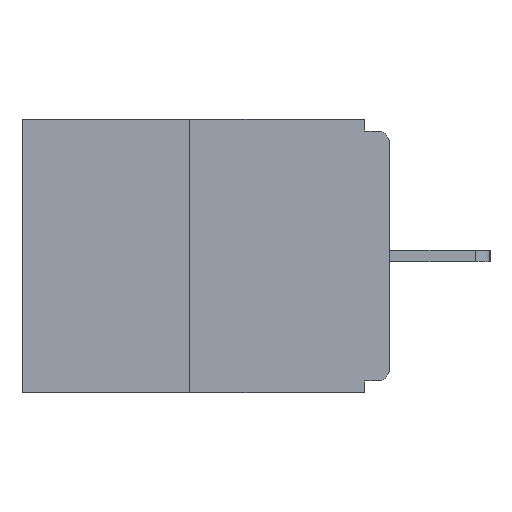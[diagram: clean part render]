
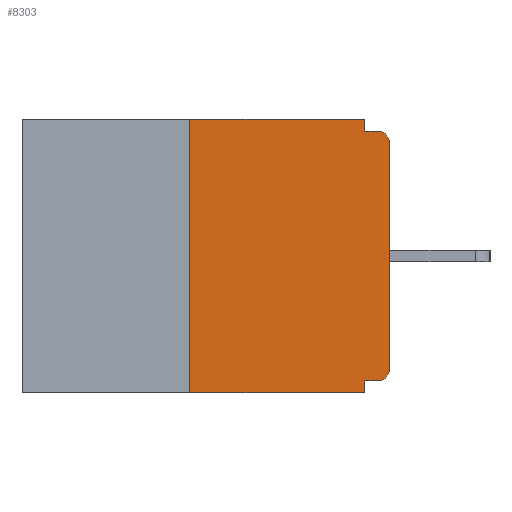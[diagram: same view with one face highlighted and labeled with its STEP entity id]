
A CAD part, left-side view. The second image highlights one B-rep face of the part: STEP entity #8303.
In plain terms, the highlighted planar face has unit normal (-1, 0, 0).
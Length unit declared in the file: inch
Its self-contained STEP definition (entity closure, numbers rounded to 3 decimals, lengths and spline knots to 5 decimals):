
#820 = VERTEX_POINT ( 'NONE', #8225 ) ;
#837 = LINE ( 'NONE', #11827, #17654 ) ;
#932 = VECTOR ( 'NONE', #15600, 39.37008 ) ;
#1601 = ORIENTED_EDGE ( 'NONE', *, *, #10227, .T. ) ;
#2636 = LINE ( 'NONE', #14006, #5194 ) ;
#3064 = EDGE_CURVE ( 'NONE', #14530, #14512, #12996, .T. ) ;
#3083 = VECTOR ( 'NONE', #16883, 39.37008 ) ;
#3139 = EDGE_CURVE ( 'NONE', #20137, #10788, #2636, .T. ) ;
#3146 = ORIENTED_EDGE ( 'NONE', *, *, #3064, .T. ) ;
#3280 = DIRECTION ( 'NONE',  ( 0., 1., 0. ) ) ;
#3359 = DIRECTION ( 'NONE',  ( 0., 0., -1. ) ) ;
#4094 = CARTESIAN_POINT ( 'NONE',  ( 0., 0.46, -0.343 ) ) ;
#4620 = ORIENTED_EDGE ( 'NONE', *, *, #8521, .F. ) ;
#5000 = CARTESIAN_POINT ( 'NONE',  ( 0., 0.015, -0.328 ) ) ;
#5194 = VECTOR ( 'NONE', #19680, 39.37008 ) ;
#5853 = ORIENTED_EDGE ( 'NONE', *, *, #8790, .F. ) ;
#5924 = CARTESIAN_POINT ( 'NONE',  ( 0., 0.015, -0.313 ) ) ;
#6240 = DIRECTION ( 'NONE',  ( -1., 0., 0. ) ) ;
#6523 = ORIENTED_EDGE ( 'NONE', *, *, #3139, .F. ) ;
#6642 = CARTESIAN_POINT ( 'NONE',  ( 0., 0.015, -0.015 ) ) ;
#6735 = LINE ( 'NONE', #13248, #15952 ) ;
#7160 = VECTOR ( 'NONE', #17291, 39.37008 ) ;
#7261 = ORIENTED_EDGE ( 'NONE', *, *, #9357, .T. ) ;
#7891 = DIRECTION ( 'NONE',  ( 1., 0., 0. ) ) ;
#8225 = CARTESIAN_POINT ( 'NONE',  ( 0., 0., -0.03 ) ) ;
#8303 = ADVANCED_FACE ( 'NONE', ( #14293 ), #17512, .F. ) ;
#8521 = EDGE_CURVE ( 'NONE', #13873, #20323, #6735, .T. ) ;
#8570 = ORIENTED_EDGE ( 'NONE', *, *, #16606, .F. ) ;
#8790 = EDGE_CURVE ( 'NONE', #14530, #13873, #19564, .T. ) ;
#8847 = CARTESIAN_POINT ( 'NONE',  ( 0., 0.015, -0.03 ) ) ;
#9051 = CARTESIAN_POINT ( 'NONE',  ( 0., 0.031, -0.015 ) ) ;
#9179 = VERTEX_POINT ( 'NONE', #11433 ) ;
#9357 = EDGE_CURVE ( 'NONE', #820, #13714, #9615, .T. ) ;
#9615 = CIRCLE ( 'NONE', #20498, 0.015 ) ;
#10192 = VECTOR ( 'NONE', #16872, 39.37008 ) ;
#10227 = EDGE_CURVE ( 'NONE', #14512, #820, #15177, .T. ) ;
#10382 = CARTESIAN_POINT ( 'NONE',  ( 0., 0., -0.015 ) ) ;
#10443 = EDGE_LOOP ( 'NONE', ( #8570, #11924, #17561, #4620, #5853, #3146, #1601, #7261, #17327, #6523 ) ) ;
#10504 = VECTOR ( 'NONE', #3280, 39.37008 ) ;
#10788 = VERTEX_POINT ( 'NONE', #9051 ) ;
#10869 = CARTESIAN_POINT ( 'NONE',  ( 0., 0.46, 0. ) ) ;
#10878 = CARTESIAN_POINT ( 'NONE',  ( 0., 0.25, -0.343 ) ) ;
#11433 = CARTESIAN_POINT ( 'NONE',  ( 0., 0.25, 0. ) ) ;
#11827 = CARTESIAN_POINT ( 'NONE',  ( 0., 0.25, 0. ) ) ;
#11924 = ORIENTED_EDGE ( 'NONE', *, *, #12956, .F. ) ;
#11957 = DIRECTION ( 'NONE',  ( 0., 0., -1. ) ) ;
#11999 = EDGE_CURVE ( 'NONE', #10788, #13714, #18597, .T. ) ;
#12189 = AXIS2_PLACEMENT_3D ( 'NONE', #16027, #7891, #3359 ) ;
#12192 = CARTESIAN_POINT ( 'NONE',  ( 0., 0., 0. ) ) ;
#12247 = DIRECTION ( 'NONE',  ( 0., 0., 1. ) ) ;
#12744 = DIRECTION ( 'NONE',  ( 0., 0., -1. ) ) ;
#12780 = CARTESIAN_POINT ( 'NONE',  ( 0., 0.031, -0.343 ) ) ;
#12956 = EDGE_CURVE ( 'NONE', #17377, #9179, #837, .T. ) ;
#12996 = CIRCLE ( 'NONE', #15727, 0.015 ) ;
#13248 = CARTESIAN_POINT ( 'NONE',  ( 0., 0.031, -0.343 ) ) ;
#13714 = VERTEX_POINT ( 'NONE', #6642 ) ;
#13737 = EDGE_CURVE ( 'NONE', #17377, #20323, #15579, .T. ) ;
#13873 = VERTEX_POINT ( 'NONE', #19099 ) ;
#14006 = CARTESIAN_POINT ( 'NONE',  ( 0., 0.031, 0. ) ) ;
#14293 = FACE_OUTER_BOUND ( 'NONE', #10443, .T. ) ;
#14512 = VERTEX_POINT ( 'NONE', #17894 ) ;
#14530 = VERTEX_POINT ( 'NONE', #5000 ) ;
#15049 = DIRECTION ( 'NONE',  ( -1., 0., 0. ) ) ;
#15177 = LINE ( 'NONE', #12192, #3083 ) ;
#15579 = LINE ( 'NONE', #4094, #10192 ) ;
#15600 = DIRECTION ( 'NONE',  ( 0., -1., 0. ) ) ;
#15727 = AXIS2_PLACEMENT_3D ( 'NONE', #5924, #6240, #12744 ) ;
#15952 = VECTOR ( 'NONE', #19749, 39.37008 ) ;
#16027 = CARTESIAN_POINT ( 'NONE',  ( 0., 0.46, 0. ) ) ;
#16269 = CARTESIAN_POINT ( 'NONE',  ( 0., 0., -0.328 ) ) ;
#16606 = EDGE_CURVE ( 'NONE', #9179, #20137, #19199, .T. ) ;
#16872 = DIRECTION ( 'NONE',  ( 0., -1., 0. ) ) ;
#16883 = DIRECTION ( 'NONE',  ( 0., 0., 1. ) ) ;
#17291 = DIRECTION ( 'NONE',  ( 0., -1., 0. ) ) ;
#17327 = ORIENTED_EDGE ( 'NONE', *, *, #11999, .F. ) ;
#17377 = VERTEX_POINT ( 'NONE', #10878 ) ;
#17512 = PLANE ( 'NONE',  #12189 ) ;
#17561 = ORIENTED_EDGE ( 'NONE', *, *, #13737, .T. ) ;
#17654 = VECTOR ( 'NONE', #12247, 39.37008 ) ;
#17894 = CARTESIAN_POINT ( 'NONE',  ( 0., 0., -0.313 ) ) ;
#18597 = LINE ( 'NONE', #10382, #932 ) ;
#19099 = CARTESIAN_POINT ( 'NONE',  ( 0., 0.031, -0.328 ) ) ;
#19199 = LINE ( 'NONE', #10869, #7160 ) ;
#19564 = LINE ( 'NONE', #16269, #10504 ) ;
#19680 = DIRECTION ( 'NONE',  ( 0., 0., -1. ) ) ;
#19749 = DIRECTION ( 'NONE',  ( 0., 0., -1. ) ) ;
#20137 = VERTEX_POINT ( 'NONE', #20559 ) ;
#20323 = VERTEX_POINT ( 'NONE', #12780 ) ;
#20498 = AXIS2_PLACEMENT_3D ( 'NONE', #8847, #15049, #11957 ) ;
#20559 = CARTESIAN_POINT ( 'NONE',  ( 0., 0.031, 0. ) ) ;
